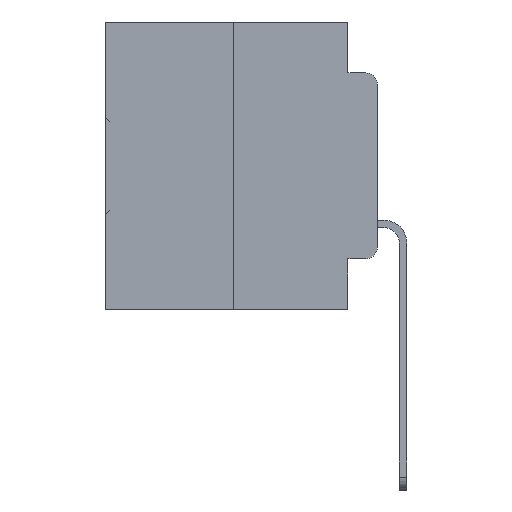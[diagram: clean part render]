
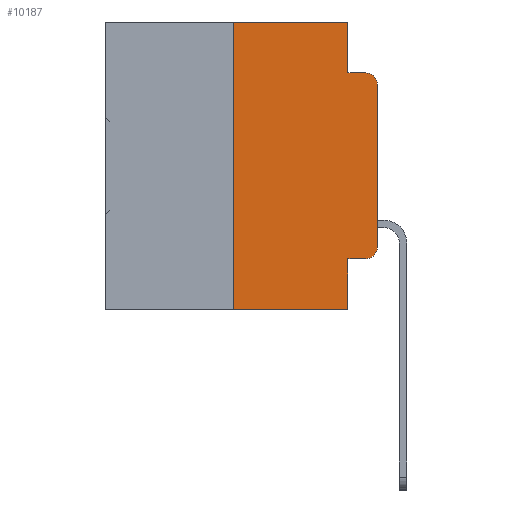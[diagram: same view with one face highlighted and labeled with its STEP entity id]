
A CAD part, left-side view. The second image highlights one B-rep face of the part: STEP entity #10187.
In plain terms, the highlighted planar face has unit normal (-1, 0, 0).
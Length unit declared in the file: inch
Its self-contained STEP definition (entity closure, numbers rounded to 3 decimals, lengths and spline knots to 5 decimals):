
#345 = CARTESIAN_POINT ( 'NONE',  ( 0., 0.051, -0.0885 ) ) ;
#409 = EDGE_LOOP ( 'NONE', ( #21120, #20226, #35584, #35399, #32151, #33676, #33635, #2269, #2481, #9780 ) ) ;
#1185 = VERTEX_POINT ( 'NONE', #8685 ) ;
#1742 = EDGE_CURVE ( 'NONE', #19039, #35429, #26853, .T. ) ;
#2269 = ORIENTED_EDGE ( 'NONE', *, *, #16320, .F. ) ;
#2481 = ORIENTED_EDGE ( 'NONE', *, *, #5041, .T. ) ;
#2712 = CIRCLE ( 'NONE', #35928, 0.02 ) ;
#3453 = AXIS2_PLACEMENT_3D ( 'NONE', #22253, #5566, #25094 ) ;
#4007 = CARTESIAN_POINT ( 'NONE',  ( 0., 0.051, 0. ) ) ;
#4876 = AXIS2_PLACEMENT_3D ( 'NONE', #8414, #22428, #5748 ) ;
#5041 = EDGE_CURVE ( 'NONE', #36158, #1185, #7727, .T. ) ;
#5070 = VECTOR ( 'NONE', #8258, 39.37008 ) ;
#5566 = DIRECTION ( 'NONE',  ( -1., 0., 0. ) ) ;
#5673 = DIRECTION ( 'NONE',  ( 0., -1., 0. ) ) ;
#5748 = DIRECTION ( 'NONE',  ( 0., 0., -1. ) ) ;
#5762 = CARTESIAN_POINT ( 'NONE',  ( 0., 0.473, 0. ) ) ;
#6767 = VECTOR ( 'NONE', #24446, 39.37008 ) ;
#7727 = LINE ( 'NONE', #13202, #21589 ) ;
#8162 = CARTESIAN_POINT ( 'NONE',  ( 0., 0.02, -0.3915 ) ) ;
#8220 = EDGE_CURVE ( 'NONE', #19039, #24808, #28436, .T. ) ;
#8234 = VERTEX_POINT ( 'NONE', #345 ) ;
#8258 = DIRECTION ( 'NONE',  ( 0., 0., 1. ) ) ;
#8414 = CARTESIAN_POINT ( 'NONE',  ( 0., 0.473, 0. ) ) ;
#8685 = CARTESIAN_POINT ( 'NONE',  ( 0., 0.02, -0.4115 ) ) ;
#9309 = EDGE_CURVE ( 'NONE', #24808, #10599, #28044, .T. ) ;
#9780 = ORIENTED_EDGE ( 'NONE', *, *, #15153, .T. ) ;
#10050 = VERTEX_POINT ( 'NONE', #24042 ) ;
#10187 = ADVANCED_FACE ( 'NONE', ( #22261 ), #14095, .F. ) ;
#10412 = LINE ( 'NONE', #4007, #32593 ) ;
#10599 = VERTEX_POINT ( 'NONE', #24244 ) ;
#10948 = DIRECTION ( 'NONE',  ( 0., 0., -1. ) ) ;
#11458 = DIRECTION ( 'NONE',  ( 0., -1., 0. ) ) ;
#12619 = VERTEX_POINT ( 'NONE', #35241 ) ;
#13098 = EDGE_CURVE ( 'NONE', #10599, #8234, #10412, .T. ) ;
#13202 = CARTESIAN_POINT ( 'NONE',  ( 0., 0.051, -0.4115 ) ) ;
#13253 = VECTOR ( 'NONE', #11458, 39.37008 ) ;
#13357 = LINE ( 'NONE', #21620, #6767 ) ;
#13945 = CIRCLE ( 'NONE', #3453, 0.02 ) ;
#14095 = PLANE ( 'NONE',  #4876 ) ;
#15153 = EDGE_CURVE ( 'NONE', #1185, #10050, #2712, .T. ) ;
#16110 = LINE ( 'NONE', #33482, #35737 ) ;
#16320 = EDGE_CURVE ( 'NONE', #36158, #35429, #13357, .T. ) ;
#16592 = CARTESIAN_POINT ( 'NONE',  ( 0., 0., 0. ) ) ;
#17930 = EDGE_CURVE ( 'NONE', #8234, #12619, #16110, .T. ) ;
#19039 = VERTEX_POINT ( 'NONE', #33410 ) ;
#20055 = CARTESIAN_POINT ( 'NONE',  ( 0., 0.25, 0. ) ) ;
#20226 = ORIENTED_EDGE ( 'NONE', *, *, #29185, .T. ) ;
#21070 = CARTESIAN_POINT ( 'NONE',  ( 0., 0.25, 0. ) ) ;
#21120 = ORIENTED_EDGE ( 'NONE', *, *, #22829, .T. ) ;
#21589 = VECTOR ( 'NONE', #32662, 39.37008 ) ;
#21620 = CARTESIAN_POINT ( 'NONE',  ( 0., 0.051, 0. ) ) ;
#21660 = CARTESIAN_POINT ( 'NONE',  ( 0., 0.051, -0.4115 ) ) ;
#21941 = CARTESIAN_POINT ( 'NONE',  ( 0., 0.473, -0.5 ) ) ;
#22253 = CARTESIAN_POINT ( 'NONE',  ( 0., 0.02, -0.1085 ) ) ;
#22261 = FACE_OUTER_BOUND ( 'NONE', #409, .T. ) ;
#22428 = DIRECTION ( 'NONE',  ( 1., 0., 0. ) ) ;
#22829 = EDGE_CURVE ( 'NONE', #10050, #34004, #27383, .T. ) ;
#22871 = DIRECTION ( 'NONE',  ( 0., 0., 1. ) ) ;
#23608 = DIRECTION ( 'NONE',  ( 0., 0., -1. ) ) ;
#24042 = CARTESIAN_POINT ( 'NONE',  ( 0., 0., -0.3915 ) ) ;
#24194 = VECTOR ( 'NONE', #24773, 39.37008 ) ;
#24244 = CARTESIAN_POINT ( 'NONE',  ( 0., 0.051, 0. ) ) ;
#24446 = DIRECTION ( 'NONE',  ( 0., 0., -1. ) ) ;
#24773 = DIRECTION ( 'NONE',  ( 0., -1., 0. ) ) ;
#24808 = VERTEX_POINT ( 'NONE', #21070 ) ;
#25094 = DIRECTION ( 'NONE',  ( 0., 0., -1. ) ) ;
#26360 = CARTESIAN_POINT ( 'NONE',  ( 0., 0.051, -0.5 ) ) ;
#26853 = LINE ( 'NONE', #21941, #24194 ) ;
#27383 = LINE ( 'NONE', #16592, #5070 ) ;
#27609 = DIRECTION ( 'NONE',  ( -1., 0., 0. ) ) ;
#28044 = LINE ( 'NONE', #5762, #13253 ) ;
#28436 = LINE ( 'NONE', #20055, #34080 ) ;
#29185 = EDGE_CURVE ( 'NONE', #34004, #12619, #13945, .T. ) ;
#32151 = ORIENTED_EDGE ( 'NONE', *, *, #9309, .F. ) ;
#32593 = VECTOR ( 'NONE', #23608, 39.37008 ) ;
#32662 = DIRECTION ( 'NONE',  ( 0., -1., 0. ) ) ;
#33410 = CARTESIAN_POINT ( 'NONE',  ( 0., 0.25, -0.5 ) ) ;
#33482 = CARTESIAN_POINT ( 'NONE',  ( 0., 0.051, -0.0885 ) ) ;
#33635 = ORIENTED_EDGE ( 'NONE', *, *, #1742, .T. ) ;
#33676 = ORIENTED_EDGE ( 'NONE', *, *, #8220, .F. ) ;
#34004 = VERTEX_POINT ( 'NONE', #34010 ) ;
#34010 = CARTESIAN_POINT ( 'NONE',  ( 0., 0., -0.1085 ) ) ;
#34080 = VECTOR ( 'NONE', #22871, 39.37008 ) ;
#35241 = CARTESIAN_POINT ( 'NONE',  ( 0., 0.02, -0.0885 ) ) ;
#35399 = ORIENTED_EDGE ( 'NONE', *, *, #13098, .F. ) ;
#35429 = VERTEX_POINT ( 'NONE', #26360 ) ;
#35584 = ORIENTED_EDGE ( 'NONE', *, *, #17930, .F. ) ;
#35737 = VECTOR ( 'NONE', #5673, 39.37008 ) ;
#35928 = AXIS2_PLACEMENT_3D ( 'NONE', #8162, #27609, #10948 ) ;
#36158 = VERTEX_POINT ( 'NONE', #21660 ) ;
